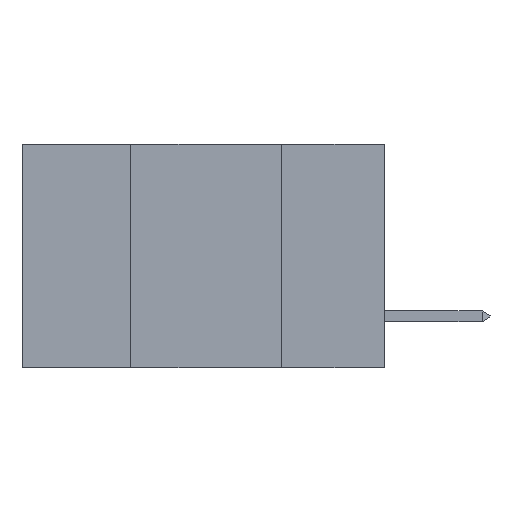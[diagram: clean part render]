
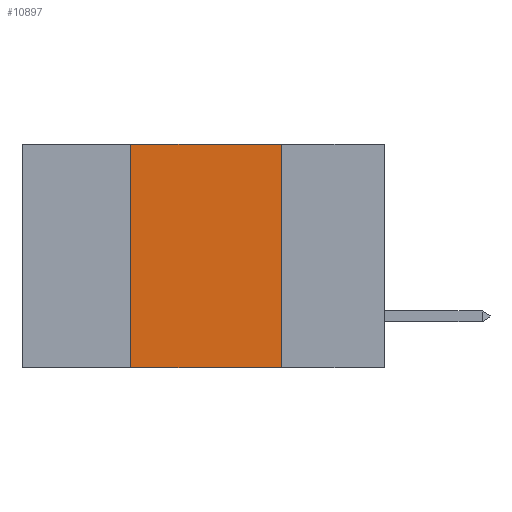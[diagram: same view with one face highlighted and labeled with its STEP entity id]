
A CAD part, left-side view. The second image highlights one B-rep face of the part: STEP entity #10897.
In plain terms, the highlighted planar face has unit normal (-1, 0, 0).
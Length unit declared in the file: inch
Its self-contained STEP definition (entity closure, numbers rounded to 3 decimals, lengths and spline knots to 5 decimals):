
#439 = VECTOR ( 'NONE', #20565, 39.37008 ) ;
#904 = CARTESIAN_POINT ( 'NONE',  ( 0., 0.42, -0.37 ) ) ;
#1450 = VERTEX_POINT ( 'NONE', #5761 ) ;
#3095 = CARTESIAN_POINT ( 'NONE',  ( 0., 0.6, -0.37 ) ) ;
#3750 = FACE_OUTER_BOUND ( 'NONE', #16157, .T. ) ;
#3855 = CARTESIAN_POINT ( 'NONE',  ( 0., 0.6, 0. ) ) ;
#3983 = DIRECTION ( 'NONE',  ( 0., 0., -1. ) ) ;
#4184 = CARTESIAN_POINT ( 'NONE',  ( 0., 0.6, 0. ) ) ;
#5671 = DIRECTION ( 'NONE',  ( 1., 0., 0. ) ) ;
#5761 = CARTESIAN_POINT ( 'NONE',  ( 0., 0.42, 0. ) ) ;
#6314 = ORIENTED_EDGE ( 'NONE', *, *, #11459, .F. ) ;
#6476 = VERTEX_POINT ( 'NONE', #20892 ) ;
#6940 = ORIENTED_EDGE ( 'NONE', *, *, #16492, .T. ) ;
#7132 = DIRECTION ( 'NONE',  ( 0., 0., -1. ) ) ;
#7486 = CARTESIAN_POINT ( 'NONE',  ( 0., 0.17, 0. ) ) ;
#7873 = VECTOR ( 'NONE', #17828, 39.37008 ) ;
#9572 = LINE ( 'NONE', #4184, #439 ) ;
#9783 = VECTOR ( 'NONE', #7132, 39.37008 ) ;
#10615 = ORIENTED_EDGE ( 'NONE', *, *, #16871, .F. ) ;
#10868 = EDGE_CURVE ( 'NONE', #21767, #1450, #12971, .T. ) ;
#10897 = ADVANCED_FACE ( 'NONE', ( #3750 ), #21797, .F. ) ;
#11459 = EDGE_CURVE ( 'NONE', #1450, #14439, #9572, .T. ) ;
#12971 = LINE ( 'NONE', #14871, #15440 ) ;
#13571 = LINE ( 'NONE', #3095, #7873 ) ;
#13844 = CARTESIAN_POINT ( 'NONE',  ( 0., 0.17, 0. ) ) ;
#14439 = VERTEX_POINT ( 'NONE', #13844 ) ;
#14871 = CARTESIAN_POINT ( 'NONE',  ( 0., 0.42, 0. ) ) ;
#15440 = VECTOR ( 'NONE', #16322, 39.37008 ) ;
#16061 = ORIENTED_EDGE ( 'NONE', *, *, #10868, .F. ) ;
#16157 = EDGE_LOOP ( 'NONE', ( #10615, #6314, #16061, #6940 ) ) ;
#16322 = DIRECTION ( 'NONE',  ( 0., 0., 1. ) ) ;
#16492 = EDGE_CURVE ( 'NONE', #21767, #6476, #13571, .T. ) ;
#16566 = LINE ( 'NONE', #7486, #9783 ) ;
#16871 = EDGE_CURVE ( 'NONE', #14439, #6476, #16566, .T. ) ;
#17828 = DIRECTION ( 'NONE',  ( 0., -1., 0. ) ) ;
#20408 = AXIS2_PLACEMENT_3D ( 'NONE', #3855, #5671, #3983 ) ;
#20565 = DIRECTION ( 'NONE',  ( 0., -1., 0. ) ) ;
#20892 = CARTESIAN_POINT ( 'NONE',  ( 0., 0.17, -0.37 ) ) ;
#21767 = VERTEX_POINT ( 'NONE', #904 ) ;
#21797 = PLANE ( 'NONE',  #20408 ) ;
